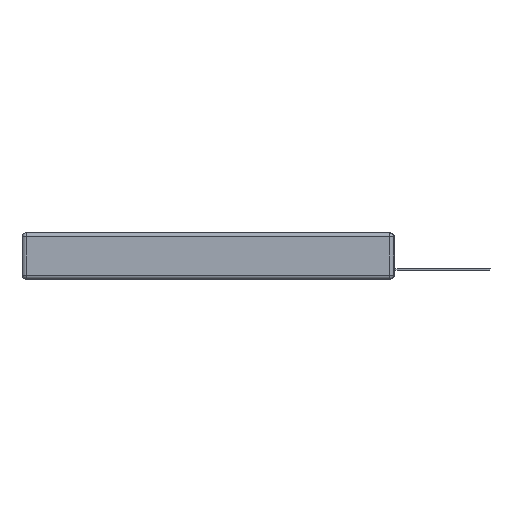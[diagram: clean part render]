
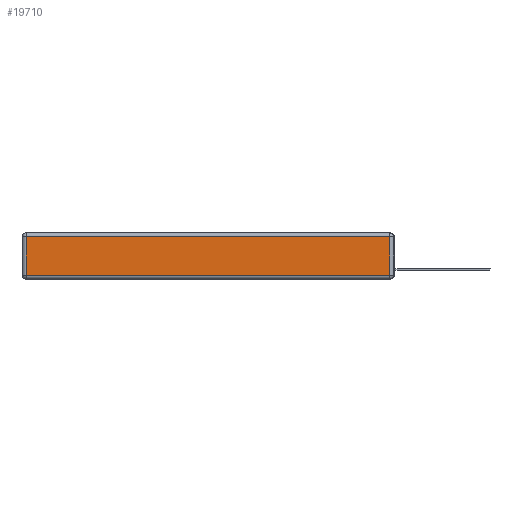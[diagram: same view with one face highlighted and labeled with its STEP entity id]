
A CAD part, left-side view. The second image highlights one B-rep face of the part: STEP entity #19710.
In plain terms, the highlighted planar face has unit normal (-1, 0, 0).
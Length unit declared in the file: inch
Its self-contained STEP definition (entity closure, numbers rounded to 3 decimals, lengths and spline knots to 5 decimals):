
#298 = EDGE_CURVE ( 'NONE', #10554, #12640, #16781, .T. ) ;
#429 = VERTEX_POINT ( 'NONE', #1500 ) ;
#626 = DIRECTION ( 'NONE',  ( -1., 0., 0. ) ) ;
#1500 = CARTESIAN_POINT ( 'NONE',  ( 0., 2.72, -0.313 ) ) ;
#2219 = FACE_OUTER_BOUND ( 'NONE', #11863, .T. ) ;
#2519 = PLANE ( 'NONE',  #11399 ) ;
#4175 = CARTESIAN_POINT ( 'NONE',  ( 0., 2.72, -0.343 ) ) ;
#5408 = CARTESIAN_POINT ( 'NONE',  ( 0., 2.75, -0.03 ) ) ;
#5801 = DIRECTION ( 'NONE',  ( 0., 0., -1. ) ) ;
#5988 = DIRECTION ( 'NONE',  ( 0., 0., 1. ) ) ;
#6796 = EDGE_CURVE ( 'NONE', #429, #10554, #18427, .T. ) ;
#6800 = CARTESIAN_POINT ( 'NONE',  ( 0., 0.03, -0.03 ) ) ;
#6863 = EDGE_CURVE ( 'NONE', #16210, #429, #19214, .T. ) ;
#7052 = CARTESIAN_POINT ( 'NONE',  ( 0., 0.03, -0.313 ) ) ;
#7506 = ORIENTED_EDGE ( 'NONE', *, *, #18410, .T. ) ;
#8308 = ORIENTED_EDGE ( 'NONE', *, *, #298, .T. ) ;
#8510 = VECTOR ( 'NONE', #9006, 39.37008 ) ;
#9006 = DIRECTION ( 'NONE',  ( 0., -1., 0. ) ) ;
#10273 = DIRECTION ( 'NONE',  ( 0., 1., 0. ) ) ;
#10554 = VERTEX_POINT ( 'NONE', #7052 ) ;
#10577 = LINE ( 'NONE', #5408, #17179 ) ;
#10841 = CARTESIAN_POINT ( 'NONE',  ( 0., 0.03, -0.343 ) ) ;
#11399 = AXIS2_PLACEMENT_3D ( 'NONE', #15183, #626, #16961 ) ;
#11863 = EDGE_LOOP ( 'NONE', ( #14337, #8308, #7506, #16897 ) ) ;
#12640 = VERTEX_POINT ( 'NONE', #6800 ) ;
#14337 = ORIENTED_EDGE ( 'NONE', *, *, #6796, .T. ) ;
#15183 = CARTESIAN_POINT ( 'NONE',  ( 0., 0., -0.343 ) ) ;
#15328 = CARTESIAN_POINT ( 'NONE',  ( 0., 2.72, -0.03 ) ) ;
#15501 = VECTOR ( 'NONE', #5988, 39.37008 ) ;
#16210 = VERTEX_POINT ( 'NONE', #15328 ) ;
#16781 = LINE ( 'NONE', #10841, #15501 ) ;
#16897 = ORIENTED_EDGE ( 'NONE', *, *, #6863, .T. ) ;
#16910 = CARTESIAN_POINT ( 'NONE',  ( 0., 0., -0.313 ) ) ;
#16961 = DIRECTION ( 'NONE',  ( 0., 0., 1. ) ) ;
#17179 = VECTOR ( 'NONE', #10273, 39.37008 ) ;
#18410 = EDGE_CURVE ( 'NONE', #12640, #16210, #10577, .T. ) ;
#18427 = LINE ( 'NONE', #16910, #8510 ) ;
#19214 = LINE ( 'NONE', #4175, #19974 ) ;
#19710 = ADVANCED_FACE ( 'NONE', ( #2219 ), #2519, .T. ) ;
#19974 = VECTOR ( 'NONE', #5801, 39.37008 ) ;
